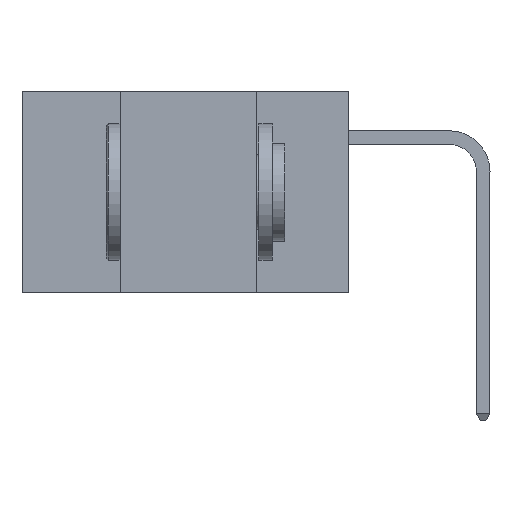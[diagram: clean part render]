
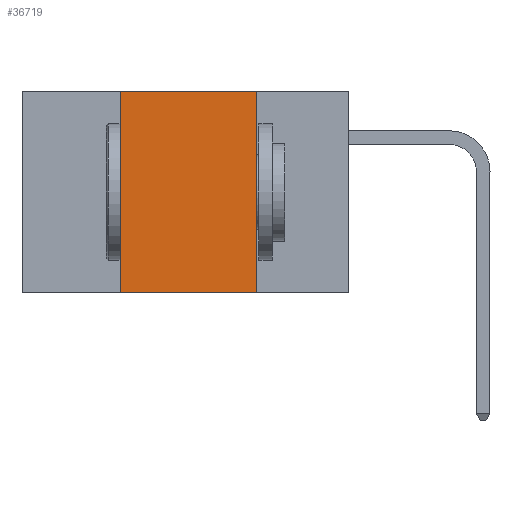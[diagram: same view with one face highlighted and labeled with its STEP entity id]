
A CAD part, left-side view. The second image highlights one B-rep face of the part: STEP entity #36719.
In plain terms, the highlighted planar face has unit normal (-1, 0, 0).
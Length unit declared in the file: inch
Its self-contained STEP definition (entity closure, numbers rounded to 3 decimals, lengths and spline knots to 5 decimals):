
#601 = LINE ( 'NONE', #32574, #34131 ) ;
#2353 = EDGE_CURVE ( 'NONE', #4329, #31714, #601, .T. ) ;
#3432 = FACE_OUTER_BOUND ( 'NONE', #13857, .T. ) ;
#4329 = VERTEX_POINT ( 'NONE', #30128 ) ;
#4530 = CARTESIAN_POINT ( 'NONE',  ( 0., 0.17, 0. ) ) ;
#5741 = ORIENTED_EDGE ( 'NONE', *, *, #2353, .F. ) ;
#8567 = ORIENTED_EDGE ( 'NONE', *, *, #12773, .T. ) ;
#9844 = DIRECTION ( 'NONE',  ( 0., 0., 1. ) ) ;
#12609 = ORIENTED_EDGE ( 'NONE', *, *, #26086, .F. ) ;
#12773 = EDGE_CURVE ( 'NONE', #19669, #19310, #29333, .T. ) ;
#13857 = EDGE_LOOP ( 'NONE', ( #12609, #5741, #21452, #8567 ) ) ;
#14661 = EDGE_CURVE ( 'NONE', #19669, #4329, #30861, .T. ) ;
#15206 = CARTESIAN_POINT ( 'NONE',  ( 0., 0.42, -0.37 ) ) ;
#16160 = DIRECTION ( 'NONE',  ( 0., 0., -1. ) ) ;
#17406 = VECTOR ( 'NONE', #16160, 39.37008 ) ;
#18274 = DIRECTION ( 'NONE',  ( 0., 0., -1. ) ) ;
#19310 = VERTEX_POINT ( 'NONE', #36319 ) ;
#19669 = VERTEX_POINT ( 'NONE', #15206 ) ;
#21452 = ORIENTED_EDGE ( 'NONE', *, *, #14661, .F. ) ;
#21779 = DIRECTION ( 'NONE',  ( 0., -1., 0. ) ) ;
#23282 = VECTOR ( 'NONE', #9844, 39.37008 ) ;
#24143 = DIRECTION ( 'NONE',  ( 0., -1., 0. ) ) ;
#24904 = LINE ( 'NONE', #4530, #17406 ) ;
#26086 = EDGE_CURVE ( 'NONE', #31714, #19310, #24904, .T. ) ;
#29333 = LINE ( 'NONE', #30117, #35847 ) ;
#29570 = PLANE ( 'NONE',  #33376 ) ;
#29622 = CARTESIAN_POINT ( 'NONE',  ( 0., 0.42, 0. ) ) ;
#30117 = CARTESIAN_POINT ( 'NONE',  ( 0., 0.6, -0.37 ) ) ;
#30128 = CARTESIAN_POINT ( 'NONE',  ( 0., 0.42, 0. ) ) ;
#30861 = LINE ( 'NONE', #29622, #23282 ) ;
#31714 = VERTEX_POINT ( 'NONE', #36560 ) ;
#32342 = CARTESIAN_POINT ( 'NONE',  ( 0., 0.6, 0. ) ) ;
#32574 = CARTESIAN_POINT ( 'NONE',  ( 0., 0.6, 0. ) ) ;
#33376 = AXIS2_PLACEMENT_3D ( 'NONE', #32342, #35169, #18274 ) ;
#34131 = VECTOR ( 'NONE', #24143, 39.37008 ) ;
#35169 = DIRECTION ( 'NONE',  ( 1., 0., 0. ) ) ;
#35847 = VECTOR ( 'NONE', #21779, 39.37008 ) ;
#36319 = CARTESIAN_POINT ( 'NONE',  ( 0., 0.17, -0.37 ) ) ;
#36560 = CARTESIAN_POINT ( 'NONE',  ( 0., 0.17, 0. ) ) ;
#36719 = ADVANCED_FACE ( 'NONE', ( #3432 ), #29570, .F. ) ;
